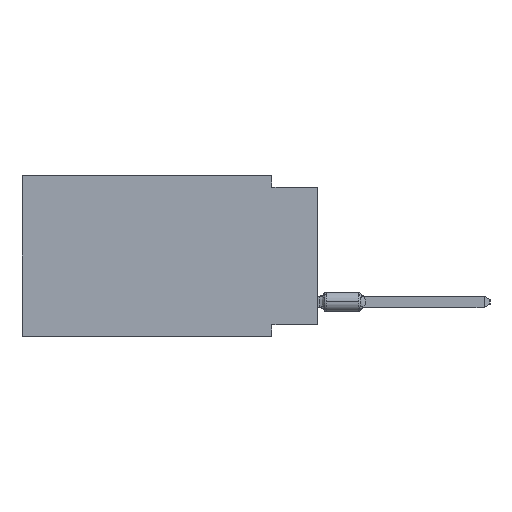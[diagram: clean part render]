
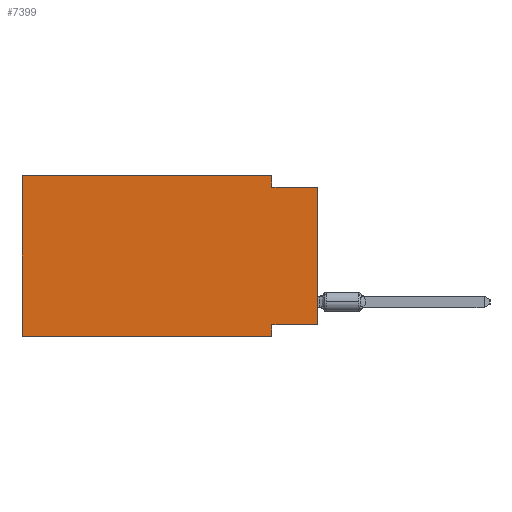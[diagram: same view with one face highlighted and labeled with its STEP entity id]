
A CAD part, left-side view. The second image highlights one B-rep face of the part: STEP entity #7399.
In plain terms, the highlighted planar face has unit normal (-1, 0, 0).
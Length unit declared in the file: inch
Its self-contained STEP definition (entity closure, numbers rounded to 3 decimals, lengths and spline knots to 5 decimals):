
#63 = DIRECTION ( 'NONE',  ( 0., -1., 0. ) ) ;
#826 = VECTOR ( 'NONE', #46091, 39.37008 ) ;
#2029 = VECTOR ( 'NONE', #33921, 39.37008 ) ;
#4108 = DIRECTION ( 'NONE',  ( 0., 1., 0. ) ) ;
#4150 = LINE ( 'NONE', #22524, #2029 ) ;
#5598 = CARTESIAN_POINT ( 'NONE',  ( 0., 0.645, 0. ) ) ;
#6221 = LINE ( 'NONE', #32770, #29860 ) ;
#6326 = VECTOR ( 'NONE', #4108, 39.37008 ) ;
#7399 = ADVANCED_FACE ( 'NONE', ( #36295 ), #20671, .F. ) ;
#8645 = CARTESIAN_POINT ( 'NONE',  ( 0., 0.1, -0.35 ) ) ;
#9138 = CARTESIAN_POINT ( 'NONE',  ( 0., 0., -0.325 ) ) ;
#9215 = DIRECTION ( 'NONE',  ( 0., 0., 1. ) ) ;
#9379 = LINE ( 'NONE', #20773, #13728 ) ;
#10539 = VERTEX_POINT ( 'NONE', #31664 ) ;
#13437 = VERTEX_POINT ( 'NONE', #9138 ) ;
#13711 = CARTESIAN_POINT ( 'NONE',  ( 0., 0.645, 0. ) ) ;
#13728 = VECTOR ( 'NONE', #24497, 39.37008 ) ;
#13865 = VERTEX_POINT ( 'NONE', #5598 ) ;
#14717 = LINE ( 'NONE', #29841, #15372 ) ;
#15372 = VECTOR ( 'NONE', #63, 39.37008 ) ;
#15595 = LINE ( 'NONE', #34438, #38592 ) ;
#16042 = EDGE_CURVE ( 'NONE', #13437, #47331, #15595, .T. ) ;
#19234 = LINE ( 'NONE', #30638, #6326 ) ;
#19579 = EDGE_CURVE ( 'NONE', #48871, #47331, #14717, .T. ) ;
#20671 = PLANE ( 'NONE',  #36665 ) ;
#20773 = CARTESIAN_POINT ( 'NONE',  ( 0., 0.645, 0. ) ) ;
#22061 = ORIENTED_EDGE ( 'NONE', *, *, #41677, .F. ) ;
#22524 = CARTESIAN_POINT ( 'NONE',  ( 0., 0.645, -0.35 ) ) ;
#24497 = DIRECTION ( 'NONE',  ( 0., -1., 0. ) ) ;
#24686 = VERTEX_POINT ( 'NONE', #30089 ) ;
#25385 = ORIENTED_EDGE ( 'NONE', *, *, #28229, .F. ) ;
#25598 = CARTESIAN_POINT ( 'NONE',  ( 0., 0., -0.025 ) ) ;
#25880 = ORIENTED_EDGE ( 'NONE', *, *, #33935, .F. ) ;
#26017 = DIRECTION ( 'NONE',  ( 0., 0., 1. ) ) ;
#28229 = EDGE_CURVE ( 'NONE', #41711, #13865, #35250, .T. ) ;
#29841 = CARTESIAN_POINT ( 'NONE',  ( 0., 0., -0.025 ) ) ;
#29860 = VECTOR ( 'NONE', #47894, 39.37008 ) ;
#30089 = CARTESIAN_POINT ( 'NONE',  ( 0., 0.1, 0. ) ) ;
#30638 = CARTESIAN_POINT ( 'NONE',  ( 0., 0., -0.325 ) ) ;
#31664 = CARTESIAN_POINT ( 'NONE',  ( 0., 0.1, -0.325 ) ) ;
#32372 = ORIENTED_EDGE ( 'NONE', *, *, #35462, .F. ) ;
#32770 = CARTESIAN_POINT ( 'NONE',  ( 0., 0.1, 0. ) ) ;
#32813 = ORIENTED_EDGE ( 'NONE', *, *, #16042, .T. ) ;
#32992 = ORIENTED_EDGE ( 'NONE', *, *, #19579, .F. ) ;
#33739 = CARTESIAN_POINT ( 'NONE',  ( 0., 0.645, -0.35 ) ) ;
#33921 = DIRECTION ( 'NONE',  ( 0., -1., 0. ) ) ;
#33935 = EDGE_CURVE ( 'NONE', #13437, #10539, #19234, .T. ) ;
#34042 = ORIENTED_EDGE ( 'NONE', *, *, #35265, .F. ) ;
#34438 = CARTESIAN_POINT ( 'NONE',  ( 0., 0., 0. ) ) ;
#35250 = LINE ( 'NONE', #46417, #48006 ) ;
#35265 = EDGE_CURVE ( 'NONE', #10539, #44053, #42119, .T. ) ;
#35462 = EDGE_CURVE ( 'NONE', #13865, #24686, #9379, .T. ) ;
#35784 = ORIENTED_EDGE ( 'NONE', *, *, #39919, .T. ) ;
#36043 = DIRECTION ( 'NONE',  ( 0., 0., -1. ) ) ;
#36295 = FACE_OUTER_BOUND ( 'NONE', #49051, .T. ) ;
#36665 = AXIS2_PLACEMENT_3D ( 'NONE', #13711, #36780, #36043 ) ;
#36780 = DIRECTION ( 'NONE',  ( 1., 0., 0. ) ) ;
#38592 = VECTOR ( 'NONE', #26017, 39.37008 ) ;
#39919 = EDGE_CURVE ( 'NONE', #41711, #44053, #4150, .T. ) ;
#41677 = EDGE_CURVE ( 'NONE', #24686, #48871, #6221, .T. ) ;
#41711 = VERTEX_POINT ( 'NONE', #33739 ) ;
#42119 = LINE ( 'NONE', #8645, #826 ) ;
#44053 = VERTEX_POINT ( 'NONE', #46669 ) ;
#46091 = DIRECTION ( 'NONE',  ( 0., 0., -1. ) ) ;
#46417 = CARTESIAN_POINT ( 'NONE',  ( 0., 0.645, 0. ) ) ;
#46669 = CARTESIAN_POINT ( 'NONE',  ( 0., 0.1, -0.35 ) ) ;
#46900 = CARTESIAN_POINT ( 'NONE',  ( 0., 0.1, -0.025 ) ) ;
#47331 = VERTEX_POINT ( 'NONE', #25598 ) ;
#47894 = DIRECTION ( 'NONE',  ( 0., 0., -1. ) ) ;
#48006 = VECTOR ( 'NONE', #9215, 39.37008 ) ;
#48871 = VERTEX_POINT ( 'NONE', #46900 ) ;
#49051 = EDGE_LOOP ( 'NONE', ( #32813, #32992, #22061, #32372, #25385, #35784, #34042, #25880 ) ) ;
